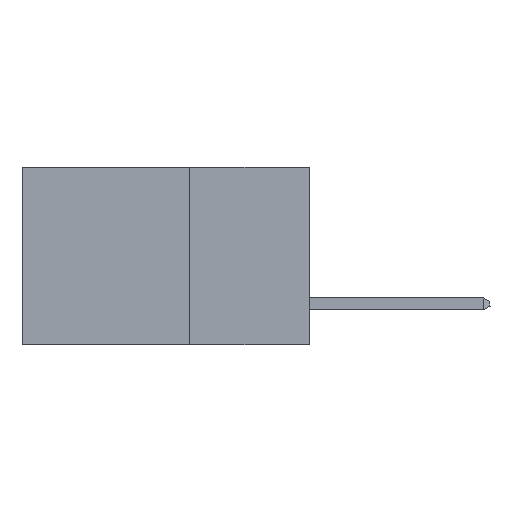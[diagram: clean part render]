
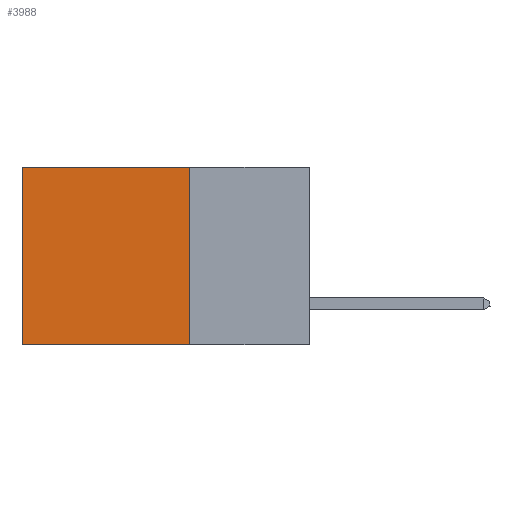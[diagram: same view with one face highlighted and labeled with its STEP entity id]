
A CAD part, left-side view. The second image highlights one B-rep face of the part: STEP entity #3988.
In plain terms, the highlighted planar face has unit normal (-1, 0, 0).
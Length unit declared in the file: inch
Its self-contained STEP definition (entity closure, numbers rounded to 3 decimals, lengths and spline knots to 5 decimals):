
#1895 = CARTESIAN_POINT ( 'NONE',  ( 0.2875, 0.6, 0. ) ) ;
#3319 = CARTESIAN_POINT ( 'NONE',  ( 0.2875, 0.25, -0.37 ) ) ;
#3988 = ADVANCED_FACE ( 'NONE', ( #20526 ), #27816, .F. ) ;
#4311 = EDGE_LOOP ( 'NONE', ( #5664, #35535, #13004, #38889 ) ) ;
#5664 = ORIENTED_EDGE ( 'NONE', *, *, #22511, .T. ) ;
#8353 = VERTEX_POINT ( 'NONE', #25929 ) ;
#8828 = VECTOR ( 'NONE', #36614, 39.37008 ) ;
#13004 = ORIENTED_EDGE ( 'NONE', *, *, #15621, .F. ) ;
#13052 = VERTEX_POINT ( 'NONE', #17474 ) ;
#13939 = VERTEX_POINT ( 'NONE', #1895 ) ;
#14553 = DIRECTION ( 'NONE',  ( 0., 0., -1. ) ) ;
#15604 = EDGE_CURVE ( 'NONE', #8353, #13939, #18475, .T. ) ;
#15621 = EDGE_CURVE ( 'NONE', #8353, #26388, #27823, .T. ) ;
#17474 = CARTESIAN_POINT ( 'NONE',  ( 0.2875, 0.6, -0.37 ) ) ;
#17490 = CARTESIAN_POINT ( 'NONE',  ( 0.2875, 0.25, -0.37 ) ) ;
#18475 = LINE ( 'NONE', #37492, #21222 ) ;
#20526 = FACE_OUTER_BOUND ( 'NONE', #4311, .T. ) ;
#21222 = VECTOR ( 'NONE', #44569, 39.37008 ) ;
#22395 = CARTESIAN_POINT ( 'NONE',  ( 0.2875, 0.6, 0. ) ) ;
#22511 = EDGE_CURVE ( 'NONE', #13939, #13052, #35338, .T. ) ;
#22893 = VECTOR ( 'NONE', #23436, 39.37008 ) ;
#23282 = CARTESIAN_POINT ( 'NONE',  ( 0.2875, 0.25, 0. ) ) ;
#23436 = DIRECTION ( 'NONE',  ( 0., 0., -1. ) ) ;
#25929 = CARTESIAN_POINT ( 'NONE',  ( 0.2875, 0.25, 0. ) ) ;
#26388 = VERTEX_POINT ( 'NONE', #17490 ) ;
#27816 = PLANE ( 'NONE',  #38288 ) ;
#27823 = LINE ( 'NONE', #23282, #22893 ) ;
#28048 = DIRECTION ( 'NONE',  ( 0., 1., 0. ) ) ;
#29404 = VECTOR ( 'NONE', #28048, 39.37008 ) ;
#32911 = EDGE_CURVE ( 'NONE', #26388, #13052, #39359, .T. ) ;
#34919 = CARTESIAN_POINT ( 'NONE',  ( 0.2875, 0.25, 0. ) ) ;
#35338 = LINE ( 'NONE', #22395, #8828 ) ;
#35535 = ORIENTED_EDGE ( 'NONE', *, *, #32911, .F. ) ;
#36614 = DIRECTION ( 'NONE',  ( 0., 0., -1. ) ) ;
#37492 = CARTESIAN_POINT ( 'NONE',  ( 0.2875, 0.25, 0. ) ) ;
#38288 = AXIS2_PLACEMENT_3D ( 'NONE', #34919, #42473, #14553 ) ;
#38889 = ORIENTED_EDGE ( 'NONE', *, *, #15604, .T. ) ;
#39359 = LINE ( 'NONE', #3319, #29404 ) ;
#42473 = DIRECTION ( 'NONE',  ( 1., 0., 0. ) ) ;
#44569 = DIRECTION ( 'NONE',  ( 0., 1., 0. ) ) ;
